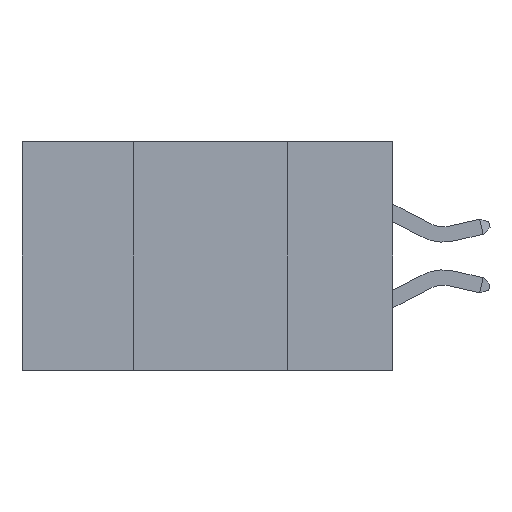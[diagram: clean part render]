
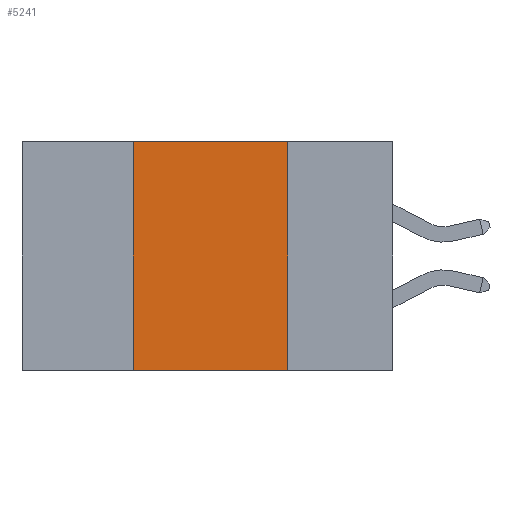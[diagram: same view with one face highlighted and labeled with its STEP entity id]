
A CAD part, left-side view. The second image highlights one B-rep face of the part: STEP entity #5241.
In plain terms, the highlighted planar face has unit normal (-1, 0, 0).
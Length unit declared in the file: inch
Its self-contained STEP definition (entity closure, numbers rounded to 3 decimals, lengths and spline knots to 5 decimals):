
#992 = CARTESIAN_POINT ( 'NONE',  ( 0., 0.42, 0. ) ) ;
#1426 = CARTESIAN_POINT ( 'NONE',  ( 0., 0.6, -0.37 ) ) ;
#1732 = LINE ( 'NONE', #992, #4099 ) ;
#2150 = DIRECTION ( 'NONE',  ( 0., -1., 0. ) ) ;
#2815 = EDGE_CURVE ( 'NONE', #5908, #4595, #6220, .T. ) ;
#2881 = LINE ( 'NONE', #6054, #10277 ) ;
#3007 = VERTEX_POINT ( 'NONE', #9262 ) ;
#3056 = VERTEX_POINT ( 'NONE', #8529 ) ;
#3061 = EDGE_CURVE ( 'NONE', #3007, #4595, #3740, .T. ) ;
#3317 = CARTESIAN_POINT ( 'NONE',  ( 0., 0.42, -0.37 ) ) ;
#3553 = PLANE ( 'NONE',  #7988 ) ;
#3586 = VECTOR ( 'NONE', #7990, 39.37008 ) ;
#3717 = DIRECTION ( 'NONE',  ( 1., 0., 0. ) ) ;
#3740 = LINE ( 'NONE', #6153, #7790 ) ;
#4099 = VECTOR ( 'NONE', #9119, 39.37008 ) ;
#4595 = VERTEX_POINT ( 'NONE', #5201 ) ;
#5201 = CARTESIAN_POINT ( 'NONE',  ( 0., 0.17, -0.37 ) ) ;
#5233 = ORIENTED_EDGE ( 'NONE', *, *, #8975, .F. ) ;
#5241 = ADVANCED_FACE ( 'NONE', ( #7548 ), #3553, .F. ) ;
#5908 = VERTEX_POINT ( 'NONE', #3317 ) ;
#6054 = CARTESIAN_POINT ( 'NONE',  ( 0., 0.6, 0. ) ) ;
#6153 = CARTESIAN_POINT ( 'NONE',  ( 0., 0.17, 0. ) ) ;
#6220 = LINE ( 'NONE', #1426, #3586 ) ;
#6806 = CARTESIAN_POINT ( 'NONE',  ( 0., 0.6, 0. ) ) ;
#7498 = EDGE_LOOP ( 'NONE', ( #8751, #9348, #5233, #8828 ) ) ;
#7548 = FACE_OUTER_BOUND ( 'NONE', #7498, .T. ) ;
#7790 = VECTOR ( 'NONE', #9359, 39.37008 ) ;
#7988 = AXIS2_PLACEMENT_3D ( 'NONE', #6806, #3717, #10056 ) ;
#7990 = DIRECTION ( 'NONE',  ( 0., -1., 0. ) ) ;
#8529 = CARTESIAN_POINT ( 'NONE',  ( 0., 0.42, 0. ) ) ;
#8751 = ORIENTED_EDGE ( 'NONE', *, *, #3061, .F. ) ;
#8828 = ORIENTED_EDGE ( 'NONE', *, *, #2815, .T. ) ;
#8975 = EDGE_CURVE ( 'NONE', #5908, #3056, #1732, .T. ) ;
#9119 = DIRECTION ( 'NONE',  ( 0., 0., 1. ) ) ;
#9262 = CARTESIAN_POINT ( 'NONE',  ( 0., 0.17, 0. ) ) ;
#9348 = ORIENTED_EDGE ( 'NONE', *, *, #9615, .F. ) ;
#9359 = DIRECTION ( 'NONE',  ( 0., 0., -1. ) ) ;
#9615 = EDGE_CURVE ( 'NONE', #3056, #3007, #2881, .T. ) ;
#10056 = DIRECTION ( 'NONE',  ( 0., 0., -1. ) ) ;
#10277 = VECTOR ( 'NONE', #2150, 39.37008 ) ;
